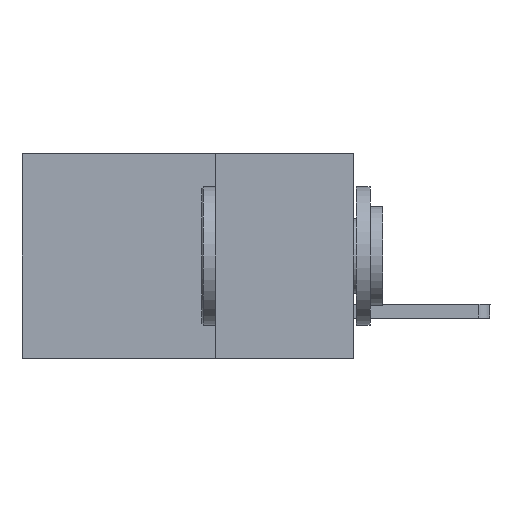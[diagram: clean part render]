
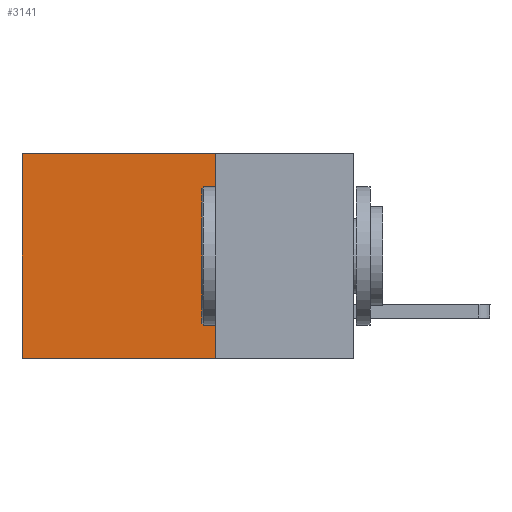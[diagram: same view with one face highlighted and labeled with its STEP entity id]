
A CAD part, left-side view. The second image highlights one B-rep face of the part: STEP entity #3141.
In plain terms, the highlighted planar face has unit normal (-1, 0, 0).
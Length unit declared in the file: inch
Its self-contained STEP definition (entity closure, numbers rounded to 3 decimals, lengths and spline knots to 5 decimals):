
#1705 = ORIENTED_EDGE ( 'NONE', *, *, #7602, .F. ) ;
#2238 = PLANE ( 'NONE',  #3308 ) ;
#2340 = VECTOR ( 'NONE', #10517, 39.37008 ) ;
#2583 = LINE ( 'NONE', #8332, #9204 ) ;
#2978 = FACE_OUTER_BOUND ( 'NONE', #5582, .T. ) ;
#3141 = ADVANCED_FACE ( 'NONE', ( #2978 ), #2238, .F. ) ;
#3308 = AXIS2_PLACEMENT_3D ( 'NONE', #4878, #5742, #9986 ) ;
#4193 = EDGE_CURVE ( 'NONE', #9819, #8273, #5678, .T. ) ;
#4424 = DIRECTION ( 'NONE',  ( 0., 1., 0. ) ) ;
#4470 = CARTESIAN_POINT ( 'NONE',  ( 0.2875, 0.25, 0. ) ) ;
#4659 = LINE ( 'NONE', #9638, #2340 ) ;
#4660 = VECTOR ( 'NONE', #8673, 39.37008 ) ;
#4676 = VERTEX_POINT ( 'NONE', #7447 ) ;
#4878 = CARTESIAN_POINT ( 'NONE',  ( 0.2875, 0.25, 0. ) ) ;
#5048 = CARTESIAN_POINT ( 'NONE',  ( 0.2875, 0.25, 0. ) ) ;
#5058 = LINE ( 'NONE', #7731, #4660 ) ;
#5582 = EDGE_LOOP ( 'NONE', ( #8683, #7929, #1705, #8163 ) ) ;
#5678 = LINE ( 'NONE', #4470, #10370 ) ;
#5742 = DIRECTION ( 'NONE',  ( 1., 0., 0. ) ) ;
#7106 = EDGE_CURVE ( 'NONE', #8273, #8287, #4659, .T. ) ;
#7447 = CARTESIAN_POINT ( 'NONE',  ( 0.2875, 0.25, -0.37 ) ) ;
#7602 = EDGE_CURVE ( 'NONE', #9819, #4676, #5058, .T. ) ;
#7731 = CARTESIAN_POINT ( 'NONE',  ( 0.2875, 0.25, 0. ) ) ;
#7929 = ORIENTED_EDGE ( 'NONE', *, *, #8492, .F. ) ;
#8163 = ORIENTED_EDGE ( 'NONE', *, *, #4193, .T. ) ;
#8273 = VERTEX_POINT ( 'NONE', #10607 ) ;
#8287 = VERTEX_POINT ( 'NONE', #10442 ) ;
#8332 = CARTESIAN_POINT ( 'NONE',  ( 0.2875, 0.25, -0.37 ) ) ;
#8492 = EDGE_CURVE ( 'NONE', #4676, #8287, #2583, .T. ) ;
#8673 = DIRECTION ( 'NONE',  ( 0., 0., -1. ) ) ;
#8683 = ORIENTED_EDGE ( 'NONE', *, *, #7106, .T. ) ;
#9204 = VECTOR ( 'NONE', #10108, 39.37008 ) ;
#9638 = CARTESIAN_POINT ( 'NONE',  ( 0.2875, 0.6, 0. ) ) ;
#9819 = VERTEX_POINT ( 'NONE', #5048 ) ;
#9986 = DIRECTION ( 'NONE',  ( 0., 0., -1. ) ) ;
#10108 = DIRECTION ( 'NONE',  ( 0., 1., 0. ) ) ;
#10370 = VECTOR ( 'NONE', #4424, 39.37008 ) ;
#10442 = CARTESIAN_POINT ( 'NONE',  ( 0.2875, 0.6, -0.37 ) ) ;
#10517 = DIRECTION ( 'NONE',  ( 0., 0., -1. ) ) ;
#10607 = CARTESIAN_POINT ( 'NONE',  ( 0.2875, 0.6, 0. ) ) ;
